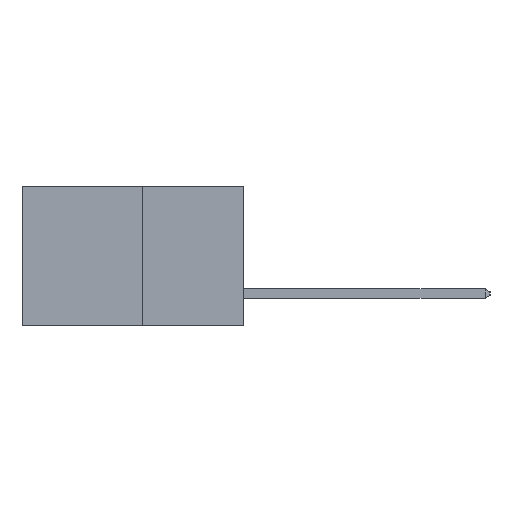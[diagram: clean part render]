
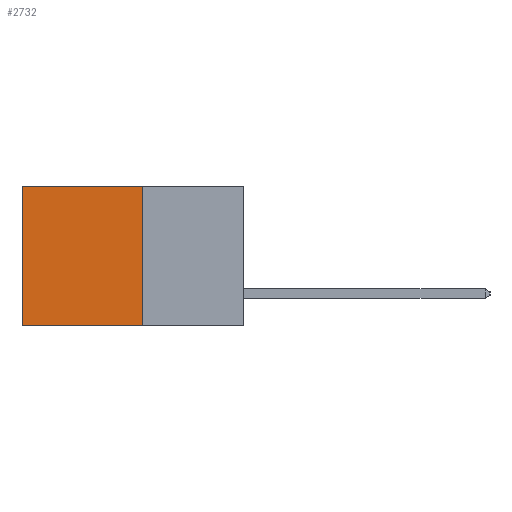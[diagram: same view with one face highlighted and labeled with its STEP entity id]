
A CAD part, left-side view. The second image highlights one B-rep face of the part: STEP entity #2732.
In plain terms, the highlighted planar face has unit normal (-1, 0, 0).
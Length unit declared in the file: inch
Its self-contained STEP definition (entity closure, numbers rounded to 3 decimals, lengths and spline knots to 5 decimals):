
#275 = VERTEX_POINT ( 'NONE', #3627 ) ;
#766 = CARTESIAN_POINT ( 'NONE',  ( 0.277, 0.27, 0. ) ) ;
#1818 = VECTOR ( 'NONE', #19253, 39.37008 ) ;
#2528 = EDGE_CURVE ( 'NONE', #4580, #12787, #17803, .T. ) ;
#2732 = ADVANCED_FACE ( 'NONE', ( #2758 ), #11158, .F. ) ;
#2758 = FACE_OUTER_BOUND ( 'NONE', #23474, .T. ) ;
#2772 = EDGE_CURVE ( 'NONE', #10421, #275, #16860, .T. ) ;
#3560 = VECTOR ( 'NONE', #14897, 39.37008 ) ;
#3615 = ORIENTED_EDGE ( 'NONE', *, *, #2528, .F. ) ;
#3627 = CARTESIAN_POINT ( 'NONE',  ( 0.277, 0.59, -0.37 ) ) ;
#4310 = CARTESIAN_POINT ( 'NONE',  ( 0.277, 0.27, -0.37 ) ) ;
#4580 = VERTEX_POINT ( 'NONE', #766 ) ;
#4722 = CARTESIAN_POINT ( 'NONE',  ( 0.277, 0.27, -0.37 ) ) ;
#5449 = EDGE_CURVE ( 'NONE', #12787, #275, #19464, .T. ) ;
#5607 = VECTOR ( 'NONE', #16088, 39.37008 ) ;
#5675 = DIRECTION ( 'NONE',  ( 0., 1., 0. ) ) ;
#8571 = CARTESIAN_POINT ( 'NONE',  ( 0.277, 0.59, -0.37 ) ) ;
#9688 = CARTESIAN_POINT ( 'NONE',  ( 0.277, 0.27, 0. ) ) ;
#10421 = VERTEX_POINT ( 'NONE', #19785 ) ;
#11158 = PLANE ( 'NONE',  #12812 ) ;
#12787 = VERTEX_POINT ( 'NONE', #22997 ) ;
#12812 = AXIS2_PLACEMENT_3D ( 'NONE', #4722, #14687, #14767 ) ;
#14687 = DIRECTION ( 'NONE',  ( 1., 0., 0. ) ) ;
#14767 = DIRECTION ( 'NONE',  ( 0., 0., -1. ) ) ;
#14897 = DIRECTION ( 'NONE',  ( 0., 1., 0. ) ) ;
#14906 = ORIENTED_EDGE ( 'NONE', *, *, #19364, .T. ) ;
#15185 = CARTESIAN_POINT ( 'NONE',  ( 0.277, 0.27, -0.37 ) ) ;
#16088 = DIRECTION ( 'NONE',  ( 0., 0., -1. ) ) ;
#16860 = LINE ( 'NONE', #8571, #5607 ) ;
#17803 = LINE ( 'NONE', #4310, #1818 ) ;
#19253 = DIRECTION ( 'NONE',  ( 0., 0., -1. ) ) ;
#19364 = EDGE_CURVE ( 'NONE', #4580, #10421, #24123, .T. ) ;
#19464 = LINE ( 'NONE', #15185, #3560 ) ;
#19785 = CARTESIAN_POINT ( 'NONE',  ( 0.277, 0.59, 0. ) ) ;
#19811 = ORIENTED_EDGE ( 'NONE', *, *, #2772, .T. ) ;
#22898 = ORIENTED_EDGE ( 'NONE', *, *, #5449, .F. ) ;
#22997 = CARTESIAN_POINT ( 'NONE',  ( 0.277, 0.27, -0.37 ) ) ;
#23474 = EDGE_LOOP ( 'NONE', ( #19811, #22898, #3615, #14906 ) ) ;
#23536 = VECTOR ( 'NONE', #5675, 39.37008 ) ;
#24123 = LINE ( 'NONE', #9688, #23536 ) ;
